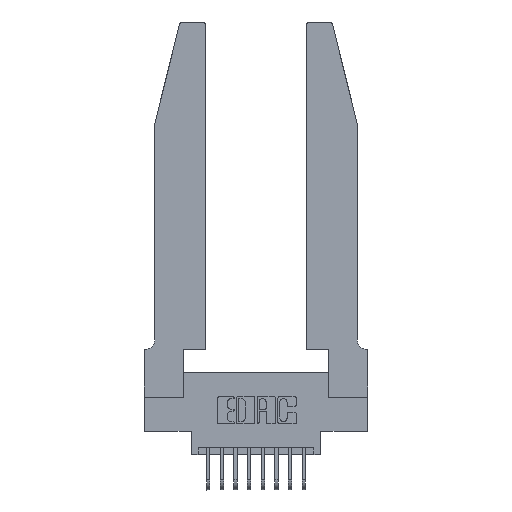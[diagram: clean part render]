
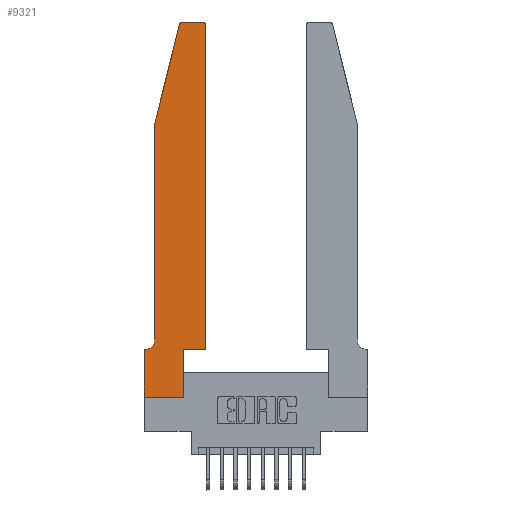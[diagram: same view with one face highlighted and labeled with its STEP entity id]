
A CAD part, top view. The second image highlights one B-rep face of the part: STEP entity #9321.
In plain terms, the highlighted planar face has unit normal (0, 0, 1).
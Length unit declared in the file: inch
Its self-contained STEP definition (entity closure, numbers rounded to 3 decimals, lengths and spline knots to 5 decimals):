
#259 = CARTESIAN_POINT ( 'NONE',  ( 0., 0.35, 0.37 ) ) ;
#390 = VECTOR ( 'NONE', #11269, 39.37008 ) ;
#573 = VERTEX_POINT ( 'NONE', #8823 ) ;
#791 = CARTESIAN_POINT ( 'NONE',  ( 0.0755, 0.35, 0.37 ) ) ;
#806 = ORIENTED_EDGE ( 'NONE', *, *, #9603, .T. ) ;
#1183 = VECTOR ( 'NONE', #9381, 39.37008 ) ;
#1645 = ORIENTED_EDGE ( 'NONE', *, *, #10321, .T. ) ;
#2627 = LINE ( 'NONE', #13393, #5796 ) ;
#2705 = LINE ( 'NONE', #15266, #8713 ) ;
#3075 = FACE_OUTER_BOUND ( 'NONE', #7870, .T. ) ;
#3258 = CIRCLE ( 'NONE', #5055, 0.07 ) ;
#3371 = CARTESIAN_POINT ( 'NONE',  ( 0.2865, 0.35, 0.37 ) ) ;
#3380 = DIRECTION ( 'NONE',  ( 0., 0., 1. ) ) ;
#3397 = CARTESIAN_POINT ( 'NONE',  ( 0.2605, 2.75, 0.37 ) ) ;
#3683 = VECTOR ( 'NONE', #11694, 39.37008 ) ;
#3799 = CARTESIAN_POINT ( 'NONE',  ( 0.0755, 2., 0.37 ) ) ;
#3900 = EDGE_CURVE ( 'NONE', #11650, #14851, #12551, .T. ) ;
#3917 = CARTESIAN_POINT ( 'NONE',  ( 0.4205, 2.72, 0.37 ) ) ;
#4169 = AXIS2_PLACEMENT_3D ( 'NONE', #3917, #12352, #5108 ) ;
#4190 = EDGE_CURVE ( 'NONE', #7316, #6645, #5542, .T. ) ;
#4424 = CARTESIAN_POINT ( 'NONE',  ( 0.4505, 0.35, 0.37 ) ) ;
#4641 = VERTEX_POINT ( 'NONE', #3371 ) ;
#4687 = LINE ( 'NONE', #12450, #390 ) ;
#4804 = CARTESIAN_POINT ( 'NONE',  ( 0.0055, 0.42, 0.37 ) ) ;
#4943 = DIRECTION ( 'NONE',  ( -0.239, -0.971, 0. ) ) ;
#5055 = AXIS2_PLACEMENT_3D ( 'NONE', #4804, #13259, #6026 ) ;
#5108 = DIRECTION ( 'NONE',  ( 1., 0., 0. ) ) ;
#5155 = VERTEX_POINT ( 'NONE', #11758 ) ;
#5373 = CARTESIAN_POINT ( 'NONE',  ( 0.4205, 2.75, 0.37 ) ) ;
#5443 = CARTESIAN_POINT ( 'NONE',  ( 0.0755, 0.42, 0.37 ) ) ;
#5513 = PLANE ( 'NONE',  #7787 ) ;
#5534 = ORIENTED_EDGE ( 'NONE', *, *, #6812, .T. ) ;
#5542 = LINE ( 'NONE', #3799, #11626 ) ;
#5726 = VERTEX_POINT ( 'NONE', #14278 ) ;
#5796 = VECTOR ( 'NONE', #4943, 39.37008 ) ;
#5834 = DIRECTION ( 'NONE',  ( 1., 0., 0. ) ) ;
#5864 = VECTOR ( 'NONE', #15195, 39.37008 ) ;
#6026 = DIRECTION ( 'NONE',  ( -1., 0., 0. ) ) ;
#6346 = CARTESIAN_POINT ( 'NONE',  ( 0.0055, 0.35, 0.37 ) ) ;
#6645 = VERTEX_POINT ( 'NONE', #5443 ) ;
#6701 = EDGE_CURVE ( 'NONE', #8639, #7320, #15115, .T. ) ;
#6729 = DIRECTION ( 'NONE',  ( 0., 0., 1. ) ) ;
#6812 = EDGE_CURVE ( 'NONE', #7884, #573, #13608, .T. ) ;
#7147 = CARTESIAN_POINT ( 'NONE',  ( 0.4505, 0.35, 0.37 ) ) ;
#7316 = VERTEX_POINT ( 'NONE', #13688 ) ;
#7320 = VERTEX_POINT ( 'NONE', #259 ) ;
#7366 = AXIS2_PLACEMENT_3D ( 'NONE', #10589, #3380, #11832 ) ;
#7787 = AXIS2_PLACEMENT_3D ( 'NONE', #11560, #6729, #15161 ) ;
#7815 = EDGE_CURVE ( 'NONE', #7320, #5726, #4687, .T. ) ;
#7870 = EDGE_LOOP ( 'NONE', ( #5534, #9376, #8141, #15568, #806, #13684, #14689, #14229, #13433, #11504, #10375, #1645 ) ) ;
#7884 = VERTEX_POINT ( 'NONE', #5373 ) ;
#8002 = VECTOR ( 'NONE', #13222, 39.37008 ) ;
#8136 = EDGE_CURVE ( 'NONE', #573, #5155, #9696, .T. ) ;
#8141 = ORIENTED_EDGE ( 'NONE', *, *, #13149, .T. ) ;
#8639 = VERTEX_POINT ( 'NONE', #6346 ) ;
#8713 = VECTOR ( 'NONE', #10462, 39.37008 ) ;
#8823 = CARTESIAN_POINT ( 'NONE',  ( 0.284, 2.75, 0.37 ) ) ;
#8959 = CARTESIAN_POINT ( 'NONE',  ( 0.4505, 0.35, 0.37 ) ) ;
#9137 = LINE ( 'NONE', #13066, #12722 ) ;
#9321 = ADVANCED_FACE ( 'NONE', ( #3075 ), #5513, .T. ) ;
#9376 = ORIENTED_EDGE ( 'NONE', *, *, #8136, .T. ) ;
#9381 = DIRECTION ( 'NONE',  ( -1., 0., 0. ) ) ;
#9389 = EDGE_CURVE ( 'NONE', #12342, #4641, #2705, .T. ) ;
#9603 = EDGE_CURVE ( 'NONE', #6645, #8639, #3258, .T. ) ;
#9696 = CIRCLE ( 'NONE', #7366, 0.03 ) ;
#10321 = EDGE_CURVE ( 'NONE', #14851, #7884, #13027, .T. ) ;
#10375 = ORIENTED_EDGE ( 'NONE', *, *, #3900, .T. ) ;
#10462 = DIRECTION ( 'NONE',  ( 0., 1., 0. ) ) ;
#10589 = CARTESIAN_POINT ( 'NONE',  ( 0.284, 2.72, 0.37 ) ) ;
#11040 = DIRECTION ( 'NONE',  ( 0., -1., 0. ) ) ;
#11269 = DIRECTION ( 'NONE',  ( 0., -1., 0. ) ) ;
#11504 = ORIENTED_EDGE ( 'NONE', *, *, #15364, .T. ) ;
#11560 = CARTESIAN_POINT ( 'NONE',  ( 0., 0.35, 0.37 ) ) ;
#11626 = VECTOR ( 'NONE', #11040, 39.37008 ) ;
#11631 = LINE ( 'NONE', #7147, #8002 ) ;
#11650 = VERTEX_POINT ( 'NONE', #8959 ) ;
#11694 = DIRECTION ( 'NONE',  ( 0., 1., 0. ) ) ;
#11758 = CARTESIAN_POINT ( 'NONE',  ( 0.25487, 2.72718, 0.37 ) ) ;
#11832 = DIRECTION ( 'NONE',  ( 1., 0., 0. ) ) ;
#12243 = CARTESIAN_POINT ( 'NONE',  ( 0.4505, 2.72, 0.37 ) ) ;
#12342 = VERTEX_POINT ( 'NONE', #12994 ) ;
#12352 = DIRECTION ( 'NONE',  ( 0., 0., 1. ) ) ;
#12450 = CARTESIAN_POINT ( 'NONE',  ( 0., 0., 0.37 ) ) ;
#12551 = LINE ( 'NONE', #4424, #3683 ) ;
#12722 = VECTOR ( 'NONE', #5834, 39.37008 ) ;
#12994 = CARTESIAN_POINT ( 'NONE',  ( 0.2865, 0., 0.37 ) ) ;
#13027 = CIRCLE ( 'NONE', #4169, 0.03 ) ;
#13066 = CARTESIAN_POINT ( 'NONE',  ( 0., 0., 0.37 ) ) ;
#13149 = EDGE_CURVE ( 'NONE', #5155, #7316, #2627, .T. ) ;
#13222 = DIRECTION ( 'NONE',  ( 1., 0., 0. ) ) ;
#13259 = DIRECTION ( 'NONE',  ( 0., 0., -1. ) ) ;
#13393 = CARTESIAN_POINT ( 'NONE',  ( 0.0755, 2., 0.37 ) ) ;
#13433 = ORIENTED_EDGE ( 'NONE', *, *, #9389, .T. ) ;
#13608 = LINE ( 'NONE', #3397, #1183 ) ;
#13684 = ORIENTED_EDGE ( 'NONE', *, *, #6701, .T. ) ;
#13688 = CARTESIAN_POINT ( 'NONE',  ( 0.0755, 2., 0.37 ) ) ;
#14229 = ORIENTED_EDGE ( 'NONE', *, *, #15272, .T. ) ;
#14278 = CARTESIAN_POINT ( 'NONE',  ( 0., 0., 0.37 ) ) ;
#14689 = ORIENTED_EDGE ( 'NONE', *, *, #7815, .T. ) ;
#14851 = VERTEX_POINT ( 'NONE', #12243 ) ;
#15115 = LINE ( 'NONE', #791, #5864 ) ;
#15161 = DIRECTION ( 'NONE',  ( 1., 0., 0. ) ) ;
#15195 = DIRECTION ( 'NONE',  ( -1., 0., 0. ) ) ;
#15266 = CARTESIAN_POINT ( 'NONE',  ( 0.2865, 0.35, 0.37 ) ) ;
#15272 = EDGE_CURVE ( 'NONE', #5726, #12342, #9137, .T. ) ;
#15364 = EDGE_CURVE ( 'NONE', #4641, #11650, #11631, .T. ) ;
#15568 = ORIENTED_EDGE ( 'NONE', *, *, #4190, .T. ) ;
